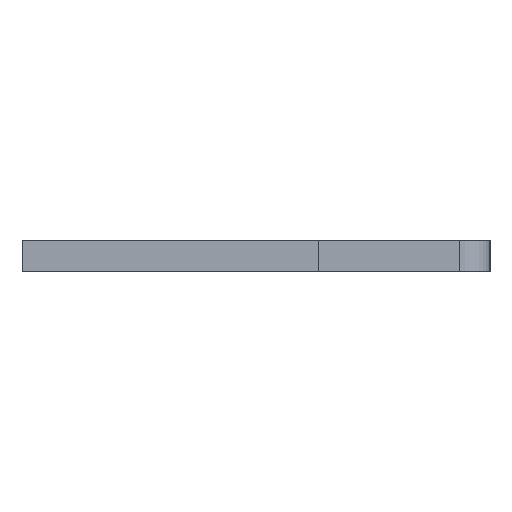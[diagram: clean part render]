
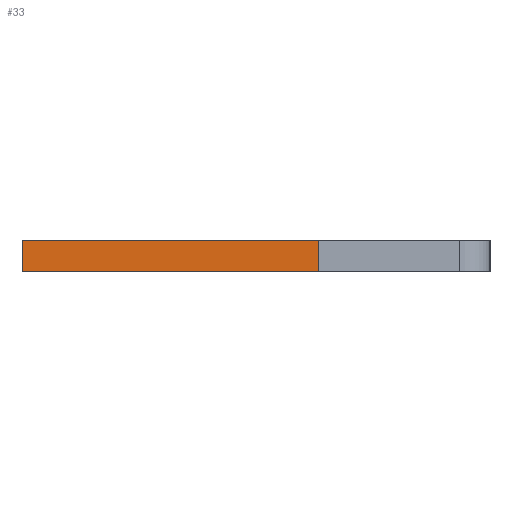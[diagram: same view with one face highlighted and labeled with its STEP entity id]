
A CAD part, left-side view. The second image highlights one B-rep face of the part: STEP entity #33.
In plain terms, the highlighted face is planar.
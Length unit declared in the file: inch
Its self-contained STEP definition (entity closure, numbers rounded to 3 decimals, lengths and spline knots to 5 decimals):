
#33 = ADVANCED_FACE ( 'NONE', ( #943 ), #1341, .F. ) ;
#56 = LINE ( 'NONE', #606, #239 ) ;
#120 = EDGE_CURVE ( 'NONE', #267, #1323, #56, .T. ) ;
#139 = CARTESIAN_POINT ( 'NONE',  ( 0.01, 0.15, -0.04 ) ) ;
#148 = CARTESIAN_POINT ( 'NONE',  ( -0.01, 0.15, -0.04 ) ) ;
#163 = DIRECTION ( 'NONE',  ( -1., 0., 0. ) ) ;
#167 = ORIENTED_EDGE ( 'NONE', *, *, #120, .T. ) ;
#168 = DIRECTION ( 'NONE',  ( 0., 1., 0. ) ) ;
#205 = VERTEX_POINT ( 'NONE', #1135 ) ;
#218 = VECTOR ( 'NONE', #1293, 39.37008 ) ;
#236 = DIRECTION ( 'NONE',  ( -1., 0., 0. ) ) ;
#239 = VECTOR ( 'NONE', #163, 39.37008 ) ;
#266 = ORIENTED_EDGE ( 'NONE', *, *, #467, .F. ) ;
#267 = VERTEX_POINT ( 'NONE', #1139 ) ;
#278 = DIRECTION ( 'NONE',  ( 0., 0., 1. ) ) ;
#307 = VERTEX_POINT ( 'NONE', #624 ) ;
#354 = VECTOR ( 'NONE', #236, 39.37008 ) ;
#386 = CARTESIAN_POINT ( 'NONE',  ( 0.01, 0.15, -0.04 ) ) ;
#458 = LINE ( 'NONE', #148, #1276 ) ;
#467 = EDGE_CURVE ( 'NONE', #205, #307, #905, .T. ) ;
#474 = EDGE_LOOP ( 'NONE', ( #767, #266, #1298, #167 ) ) ;
#485 = DIRECTION ( 'NONE',  ( 1., 0., 0. ) ) ;
#586 = LINE ( 'NONE', #139, #218 ) ;
#606 = CARTESIAN_POINT ( 'NONE',  ( 0.01, -0.04, -0.04 ) ) ;
#624 = CARTESIAN_POINT ( 'NONE',  ( -0.01, 0.15, -0.04 ) ) ;
#767 = ORIENTED_EDGE ( 'NONE', *, *, #1136, .T. ) ;
#786 = AXIS2_PLACEMENT_3D ( 'NONE', #386, #278, #485 ) ;
#801 = EDGE_CURVE ( 'NONE', #267, #205, #586, .T. ) ;
#905 = LINE ( 'NONE', #1061, #354 ) ;
#943 = FACE_OUTER_BOUND ( 'NONE', #474, .T. ) ;
#990 = CARTESIAN_POINT ( 'NONE',  ( -0.01, -0.04, -0.04 ) ) ;
#1061 = CARTESIAN_POINT ( 'NONE',  ( 0.01, 0.15, -0.04 ) ) ;
#1135 = CARTESIAN_POINT ( 'NONE',  ( 0.01, 0.15, -0.04 ) ) ;
#1136 = EDGE_CURVE ( 'NONE', #1323, #307, #458, .T. ) ;
#1139 = CARTESIAN_POINT ( 'NONE',  ( 0.01, -0.04, -0.04 ) ) ;
#1276 = VECTOR ( 'NONE', #168, 39.37008 ) ;
#1293 = DIRECTION ( 'NONE',  ( 0., 1., 0. ) ) ;
#1298 = ORIENTED_EDGE ( 'NONE', *, *, #801, .F. ) ;
#1323 = VERTEX_POINT ( 'NONE', #990 ) ;
#1341 = PLANE ( 'NONE',  #786 ) ;
